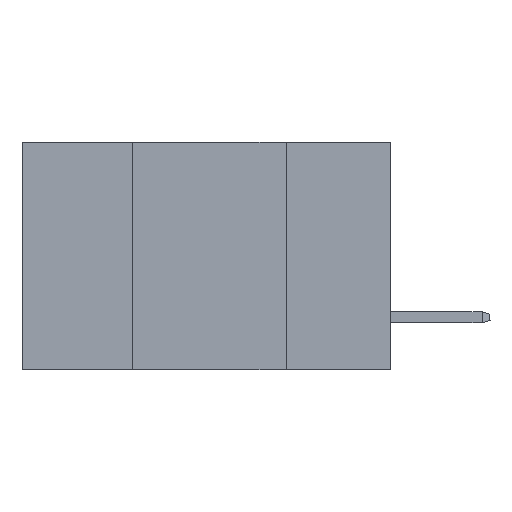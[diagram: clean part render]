
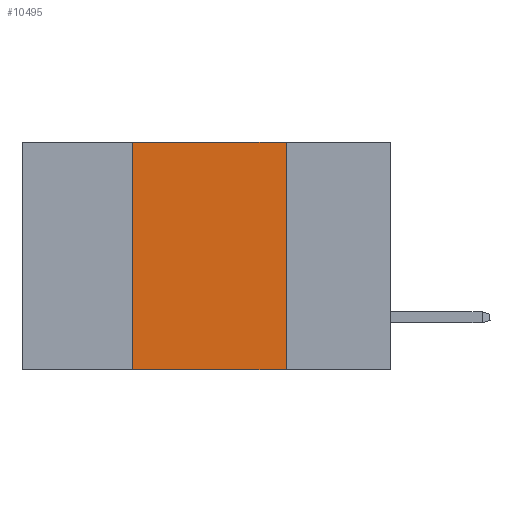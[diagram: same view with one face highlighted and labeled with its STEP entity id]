
A CAD part, left-side view. The second image highlights one B-rep face of the part: STEP entity #10495.
In plain terms, the highlighted planar face has unit normal (-1, 0, 0).
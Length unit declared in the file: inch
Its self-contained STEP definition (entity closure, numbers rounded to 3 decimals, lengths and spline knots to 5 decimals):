
#206 = EDGE_CURVE ( 'NONE', #22766, #24966, #38976, .T. ) ;
#983 = VECTOR ( 'NONE', #25080, 39.37008 ) ;
#2280 = VECTOR ( 'NONE', #30546, 39.37008 ) ;
#3059 = VERTEX_POINT ( 'NONE', #8591 ) ;
#3259 = LINE ( 'NONE', #24682, #2280 ) ;
#3839 = CARTESIAN_POINT ( 'NONE',  ( 0., 0.6, -0.37 ) ) ;
#7439 = DIRECTION ( 'NONE',  ( 0., -1., 0. ) ) ;
#8591 = CARTESIAN_POINT ( 'NONE',  ( 0., 0.17, -0.37 ) ) ;
#10495 = ADVANCED_FACE ( 'NONE', ( #14782 ), #20598, .F. ) ;
#14018 = VECTOR ( 'NONE', #7439, 39.37008 ) ;
#14134 = CARTESIAN_POINT ( 'NONE',  ( 0., 0.6, 0. ) ) ;
#14542 = CARTESIAN_POINT ( 'NONE',  ( 0., 0.6, 0. ) ) ;
#14673 = DIRECTION ( 'NONE',  ( 0., 0., -1. ) ) ;
#14782 = FACE_OUTER_BOUND ( 'NONE', #33498, .T. ) ;
#18166 = LINE ( 'NONE', #3839, #983 ) ;
#19144 = ORIENTED_EDGE ( 'NONE', *, *, #206, .F. ) ;
#20527 = ORIENTED_EDGE ( 'NONE', *, *, #22793, .F. ) ;
#20598 = PLANE ( 'NONE',  #39007 ) ;
#21963 = VERTEX_POINT ( 'NONE', #31383 ) ;
#22766 = VERTEX_POINT ( 'NONE', #31964 ) ;
#22793 = EDGE_CURVE ( 'NONE', #24966, #3059, #31013, .T. ) ;
#23050 = VECTOR ( 'NONE', #32218, 39.37008 ) ;
#24682 = CARTESIAN_POINT ( 'NONE',  ( 0., 0.42, 0. ) ) ;
#24966 = VERTEX_POINT ( 'NONE', #30794 ) ;
#25080 = DIRECTION ( 'NONE',  ( 0., -1., 0. ) ) ;
#29228 = CARTESIAN_POINT ( 'NONE',  ( 0., 0.17, 0. ) ) ;
#29940 = ORIENTED_EDGE ( 'NONE', *, *, #38479, .F. ) ;
#30546 = DIRECTION ( 'NONE',  ( 0., 0., 1. ) ) ;
#30794 = CARTESIAN_POINT ( 'NONE',  ( 0., 0.17, 0. ) ) ;
#31013 = LINE ( 'NONE', #29228, #23050 ) ;
#31383 = CARTESIAN_POINT ( 'NONE',  ( 0., 0.42, -0.37 ) ) ;
#31964 = CARTESIAN_POINT ( 'NONE',  ( 0., 0.42, 0. ) ) ;
#32218 = DIRECTION ( 'NONE',  ( 0., 0., -1. ) ) ;
#32689 = DIRECTION ( 'NONE',  ( 1., 0., 0. ) ) ;
#33498 = EDGE_LOOP ( 'NONE', ( #20527, #19144, #29940, #37979 ) ) ;
#35678 = EDGE_CURVE ( 'NONE', #21963, #3059, #18166, .T. ) ;
#37979 = ORIENTED_EDGE ( 'NONE', *, *, #35678, .T. ) ;
#38479 = EDGE_CURVE ( 'NONE', #21963, #22766, #3259, .T. ) ;
#38976 = LINE ( 'NONE', #14134, #14018 ) ;
#39007 = AXIS2_PLACEMENT_3D ( 'NONE', #14542, #32689, #14673 ) ;
